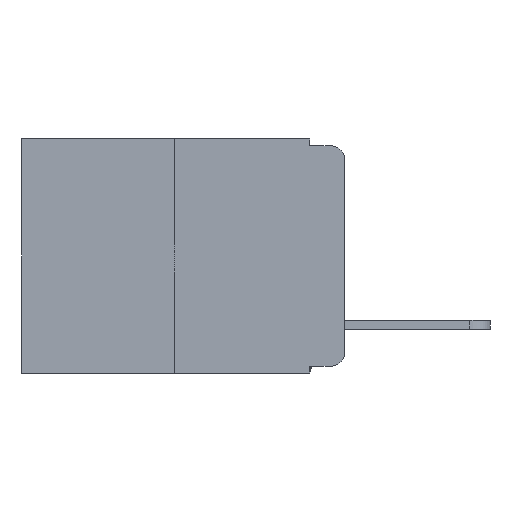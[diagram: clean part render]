
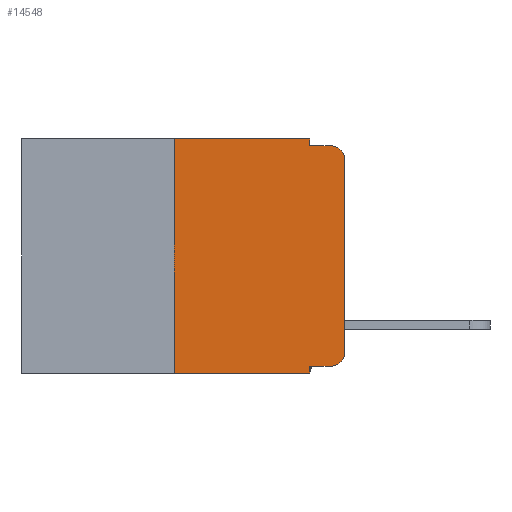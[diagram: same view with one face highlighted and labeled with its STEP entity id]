
A CAD part, left-side view. The second image highlights one B-rep face of the part: STEP entity #14548.
In plain terms, the highlighted planar face has unit normal (-1, 0, 0).
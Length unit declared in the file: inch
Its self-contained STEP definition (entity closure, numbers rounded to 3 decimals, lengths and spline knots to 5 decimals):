
#243 = VECTOR ( 'NONE', #13124, 39.37008 ) ;
#245 = ORIENTED_EDGE ( 'NONE', *, *, #9357, .F. ) ;
#431 = CARTESIAN_POINT ( 'NONE',  ( 0., 0.473, -0.343 ) ) ;
#524 = ORIENTED_EDGE ( 'NONE', *, *, #9267, .F. ) ;
#825 = ORIENTED_EDGE ( 'NONE', *, *, #8764, .T. ) ;
#1100 = ORIENTED_EDGE ( 'NONE', *, *, #8237, .F. ) ;
#1217 = AXIS2_PLACEMENT_3D ( 'NONE', #17890, #8512, #19279 ) ;
#1787 = VERTEX_POINT ( 'NONE', #19630 ) ;
#1995 = PLANE ( 'NONE',  #1217 ) ;
#2450 = CARTESIAN_POINT ( 'NONE',  ( 0., 0.051, 0. ) ) ;
#2620 = FACE_OUTER_BOUND ( 'NONE', #7480, .T. ) ;
#3288 = LINE ( 'NONE', #14381, #11188 ) ;
#3779 = VECTOR ( 'NONE', #13102, 39.37008 ) ;
#4261 = LINE ( 'NONE', #13182, #243 ) ;
#4288 = LINE ( 'NONE', #15076, #8551 ) ;
#4329 = CARTESIAN_POINT ( 'NONE',  ( 0., 0.051, -0.343 ) ) ;
#5029 = CARTESIAN_POINT ( 'NONE',  ( 0., 0.051, -0.333 ) ) ;
#5303 = ORIENTED_EDGE ( 'NONE', *, *, #9360, .F. ) ;
#5499 = CARTESIAN_POINT ( 'NONE',  ( 0., 0., -0.03 ) ) ;
#6515 = CARTESIAN_POINT ( 'NONE',  ( 0., 0., -0.313 ) ) ;
#6571 = VERTEX_POINT ( 'NONE', #6515 ) ;
#7093 = CIRCLE ( 'NONE', #18428, 0.02 ) ;
#7480 = EDGE_LOOP ( 'NONE', ( #15179, #8299, #524, #17623, #1100, #245, #825, #5303, #11422, #12700 ) ) ;
#7593 = CIRCLE ( 'NONE', #12143, 0.02 ) ;
#7898 = CARTESIAN_POINT ( 'NONE',  ( 0., 0.473, 0. ) ) ;
#8003 = VERTEX_POINT ( 'NONE', #4329 ) ;
#8062 = LINE ( 'NONE', #13039, #15951 ) ;
#8237 = EDGE_CURVE ( 'NONE', #17760, #20380, #10259, .T. ) ;
#8299 = ORIENTED_EDGE ( 'NONE', *, *, #9262, .T. ) ;
#8512 = DIRECTION ( 'NONE',  ( 1., 0., 0. ) ) ;
#8534 = VERTEX_POINT ( 'NONE', #8722 ) ;
#8551 = VECTOR ( 'NONE', #15505, 39.37008 ) ;
#8722 = CARTESIAN_POINT ( 'NONE',  ( 0., 0.02, -0.01 ) ) ;
#8764 = EDGE_CURVE ( 'NONE', #1787, #8003, #18757, .T. ) ;
#8994 = LINE ( 'NONE', #13717, #16921 ) ;
#9234 = EDGE_CURVE ( 'NONE', #6571, #14970, #4288, .T. ) ;
#9262 = EDGE_CURVE ( 'NONE', #14970, #8534, #7593, .T. ) ;
#9267 = EDGE_CURVE ( 'NONE', #16382, #8534, #3288, .T. ) ;
#9321 = EDGE_CURVE ( 'NONE', #20380, #16382, #8994, .T. ) ;
#9357 = EDGE_CURVE ( 'NONE', #1787, #17760, #4261, .T. ) ;
#9360 = EDGE_CURVE ( 'NONE', #14483, #8003, #16456, .T. ) ;
#9361 = EDGE_CURVE ( 'NONE', #14483, #14078, #8062, .T. ) ;
#9419 = EDGE_CURVE ( 'NONE', #14078, #6571, #7093, .T. ) ;
#9783 = VECTOR ( 'NONE', #19919, 39.37008 ) ;
#10259 = LINE ( 'NONE', #7898, #9783 ) ;
#11188 = VECTOR ( 'NONE', #14542, 39.37008 ) ;
#11297 = CARTESIAN_POINT ( 'NONE',  ( 0., 0.25, 0. ) ) ;
#11422 = ORIENTED_EDGE ( 'NONE', *, *, #9361, .T. ) ;
#12143 = AXIS2_PLACEMENT_3D ( 'NONE', #14358, #14341, #14334 ) ;
#12548 = DIRECTION ( 'NONE',  ( 0., 0., -1. ) ) ;
#12553 = CARTESIAN_POINT ( 'NONE',  ( 0., 0.02, -0.333 ) ) ;
#12555 = DIRECTION ( 'NONE',  ( -1., 0., 0. ) ) ;
#12565 = CARTESIAN_POINT ( 'NONE',  ( 0., 0.02, -0.313 ) ) ;
#12700 = ORIENTED_EDGE ( 'NONE', *, *, #9419, .T. ) ;
#12971 = DIRECTION ( 'NONE',  ( 0., -1., 0. ) ) ;
#13039 = CARTESIAN_POINT ( 'NONE',  ( 0., 0.051, -0.333 ) ) ;
#13102 = DIRECTION ( 'NONE',  ( 0., 0., -1. ) ) ;
#13124 = DIRECTION ( 'NONE',  ( 0., 0., 1. ) ) ;
#13182 = CARTESIAN_POINT ( 'NONE',  ( 0., 0.25, 0. ) ) ;
#13204 = CARTESIAN_POINT ( 'NONE',  ( 0., 0.051, 0. ) ) ;
#13363 = DIRECTION ( 'NONE',  ( 0., 0., -1. ) ) ;
#13717 = CARTESIAN_POINT ( 'NONE',  ( 0., 0.051, 0. ) ) ;
#14078 = VERTEX_POINT ( 'NONE', #12553 ) ;
#14334 = DIRECTION ( 'NONE',  ( 0., 0., -1. ) ) ;
#14341 = DIRECTION ( 'NONE',  ( -1., 0., 0. ) ) ;
#14358 = CARTESIAN_POINT ( 'NONE',  ( 0., 0.02, -0.03 ) ) ;
#14381 = CARTESIAN_POINT ( 'NONE',  ( 0., 0.051, -0.01 ) ) ;
#14483 = VERTEX_POINT ( 'NONE', #5029 ) ;
#14542 = DIRECTION ( 'NONE',  ( 0., -1., 0. ) ) ;
#14548 = ADVANCED_FACE ( 'NONE', ( #2620 ), #1995, .F. ) ;
#14738 = VECTOR ( 'NONE', #20268, 39.37008 ) ;
#14970 = VERTEX_POINT ( 'NONE', #5499 ) ;
#15076 = CARTESIAN_POINT ( 'NONE',  ( 0., 0., 0. ) ) ;
#15179 = ORIENTED_EDGE ( 'NONE', *, *, #9234, .T. ) ;
#15505 = DIRECTION ( 'NONE',  ( 0., 0., 1. ) ) ;
#15951 = VECTOR ( 'NONE', #12971, 39.37008 ) ;
#16382 = VERTEX_POINT ( 'NONE', #18994 ) ;
#16456 = LINE ( 'NONE', #13204, #3779 ) ;
#16921 = VECTOR ( 'NONE', #13363, 39.37008 ) ;
#17623 = ORIENTED_EDGE ( 'NONE', *, *, #9321, .F. ) ;
#17760 = VERTEX_POINT ( 'NONE', #11297 ) ;
#17890 = CARTESIAN_POINT ( 'NONE',  ( 0., 0.473, 0. ) ) ;
#18428 = AXIS2_PLACEMENT_3D ( 'NONE', #12565, #12555, #12548 ) ;
#18757 = LINE ( 'NONE', #431, #14738 ) ;
#18994 = CARTESIAN_POINT ( 'NONE',  ( 0., 0.051, -0.01 ) ) ;
#19279 = DIRECTION ( 'NONE',  ( 0., 0., -1. ) ) ;
#19630 = CARTESIAN_POINT ( 'NONE',  ( 0., 0.25, -0.343 ) ) ;
#19919 = DIRECTION ( 'NONE',  ( 0., -1., 0. ) ) ;
#20268 = DIRECTION ( 'NONE',  ( 0., -1., 0. ) ) ;
#20380 = VERTEX_POINT ( 'NONE', #2450 ) ;
